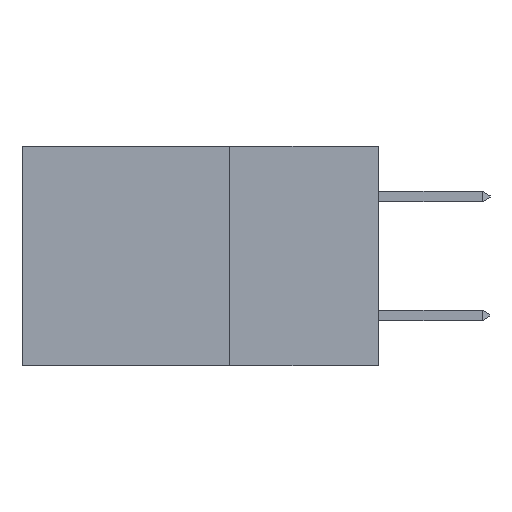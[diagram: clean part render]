
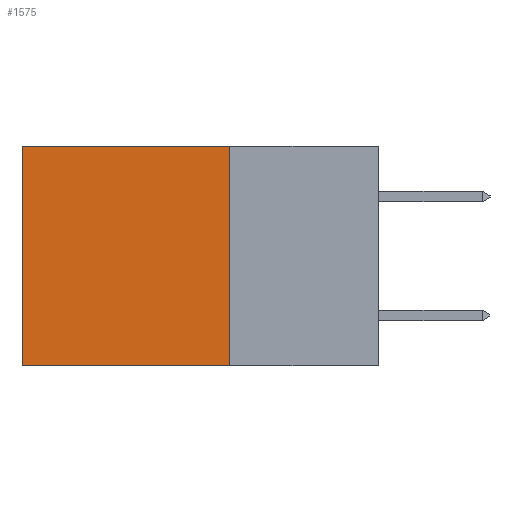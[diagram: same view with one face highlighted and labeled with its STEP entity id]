
A CAD part, left-side view. The second image highlights one B-rep face of the part: STEP entity #1575.
In plain terms, the highlighted planar face has unit normal (-1, 0, 0).
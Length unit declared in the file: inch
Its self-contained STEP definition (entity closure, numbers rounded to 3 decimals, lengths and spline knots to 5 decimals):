
#4 = VERTEX_POINT ( 'NONE', #10444 ) ;
#1197 = DIRECTION ( 'NONE',  ( 0., 1., 0. ) ) ;
#1413 = VECTOR ( 'NONE', #1197, 39.37008 ) ;
#1449 = EDGE_CURVE ( 'NONE', #11707, #10035, #6014, .T. ) ;
#1575 = ADVANCED_FACE ( 'NONE', ( #14899 ), #6300, .F. ) ;
#1935 = VECTOR ( 'NONE', #8837, 39.37008 ) ;
#2015 = EDGE_CURVE ( 'NONE', #16600, #4, #8371, .T. ) ;
#2122 = CARTESIAN_POINT ( 'NONE',  ( 0.298, 0.6, 0. ) ) ;
#2397 = VECTOR ( 'NONE', #9884, 39.37008 ) ;
#3441 = ORIENTED_EDGE ( 'NONE', *, *, #13737, .T. ) ;
#3650 = EDGE_CURVE ( 'NONE', #10035, #4, #14749, .T. ) ;
#3789 = ORIENTED_EDGE ( 'NONE', *, *, #2015, .T. ) ;
#5380 = CARTESIAN_POINT ( 'NONE',  ( 0.298, 0.25, 0. ) ) ;
#5547 = AXIS2_PLACEMENT_3D ( 'NONE', #5380, #9970, #15576 ) ;
#5823 = CARTESIAN_POINT ( 'NONE',  ( 0.298, 0.6, 0. ) ) ;
#6014 = LINE ( 'NONE', #10480, #2397 ) ;
#6300 = PLANE ( 'NONE',  #5547 ) ;
#7649 = CARTESIAN_POINT ( 'NONE',  ( 0.298, 0.25, -0.37 ) ) ;
#8371 = LINE ( 'NONE', #5823, #14884 ) ;
#8796 = LINE ( 'NONE', #16518, #1935 ) ;
#8837 = DIRECTION ( 'NONE',  ( 0., 1., 0. ) ) ;
#9808 = ORIENTED_EDGE ( 'NONE', *, *, #1449, .F. ) ;
#9884 = DIRECTION ( 'NONE',  ( 0., 0., -1. ) ) ;
#9970 = DIRECTION ( 'NONE',  ( 1., 0., 0. ) ) ;
#10035 = VERTEX_POINT ( 'NONE', #7649 ) ;
#10444 = CARTESIAN_POINT ( 'NONE',  ( 0.298, 0.6, -0.37 ) ) ;
#10480 = CARTESIAN_POINT ( 'NONE',  ( 0.298, 0.25, 0. ) ) ;
#11707 = VERTEX_POINT ( 'NONE', #16375 ) ;
#11989 = EDGE_LOOP ( 'NONE', ( #3789, #16971, #9808, #3441 ) ) ;
#13737 = EDGE_CURVE ( 'NONE', #11707, #16600, #8796, .T. ) ;
#14749 = LINE ( 'NONE', #16951, #1413 ) ;
#14884 = VECTOR ( 'NONE', #16482, 39.37008 ) ;
#14899 = FACE_OUTER_BOUND ( 'NONE', #11989, .T. ) ;
#15576 = DIRECTION ( 'NONE',  ( 0., 0., -1. ) ) ;
#16375 = CARTESIAN_POINT ( 'NONE',  ( 0.298, 0.25, 0. ) ) ;
#16482 = DIRECTION ( 'NONE',  ( 0., 0., -1. ) ) ;
#16518 = CARTESIAN_POINT ( 'NONE',  ( 0.298, 0.25, 0. ) ) ;
#16600 = VERTEX_POINT ( 'NONE', #2122 ) ;
#16951 = CARTESIAN_POINT ( 'NONE',  ( 0.298, 0.25, -0.37 ) ) ;
#16971 = ORIENTED_EDGE ( 'NONE', *, *, #3650, .F. ) ;
